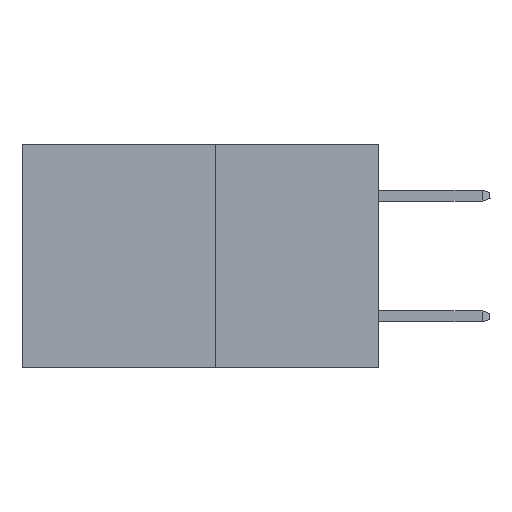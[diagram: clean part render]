
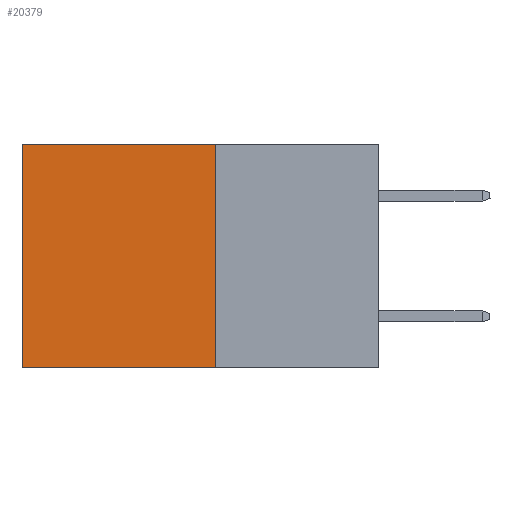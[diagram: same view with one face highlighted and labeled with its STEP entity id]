
A CAD part, left-side view. The second image highlights one B-rep face of the part: STEP entity #20379.
In plain terms, the highlighted planar face has unit normal (-1, 0, 0).
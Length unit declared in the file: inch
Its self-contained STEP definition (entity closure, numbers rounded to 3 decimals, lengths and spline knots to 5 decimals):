
#236 = LINE ( 'NONE', #17223, #17540 ) ;
#738 = ORIENTED_EDGE ( 'NONE', *, *, #6208, .T. ) ;
#1048 = DIRECTION ( 'NONE',  ( 1., 0., 0. ) ) ;
#1437 = CARTESIAN_POINT ( 'NONE',  ( 0.277, 0.59, 0. ) ) ;
#1688 = LINE ( 'NONE', #9182, #18836 ) ;
#2247 = VERTEX_POINT ( 'NONE', #9369 ) ;
#2275 = FACE_OUTER_BOUND ( 'NONE', #19413, .T. ) ;
#2917 = CARTESIAN_POINT ( 'NONE',  ( 0.277, 0.27, -0.37 ) ) ;
#3136 = VERTEX_POINT ( 'NONE', #7592 ) ;
#3161 = ORIENTED_EDGE ( 'NONE', *, *, #16661, .F. ) ;
#4608 = DIRECTION ( 'NONE',  ( 0., 1., 0. ) ) ;
#5179 = VERTEX_POINT ( 'NONE', #1437 ) ;
#6208 = EDGE_CURVE ( 'NONE', #5179, #2247, #236, .T. ) ;
#6467 = EDGE_CURVE ( 'NONE', #13673, #2247, #15794, .T. ) ;
#7592 = CARTESIAN_POINT ( 'NONE',  ( 0.277, 0.27, 0. ) ) ;
#7734 = DIRECTION ( 'NONE',  ( 0., 1., 0. ) ) ;
#8512 = VECTOR ( 'NONE', #4608, 39.37008 ) ;
#9182 = CARTESIAN_POINT ( 'NONE',  ( 0.277, 0.27, -0.37 ) ) ;
#9369 = CARTESIAN_POINT ( 'NONE',  ( 0.277, 0.59, -0.37 ) ) ;
#10660 = DIRECTION ( 'NONE',  ( 0., 0., -1. ) ) ;
#11067 = CARTESIAN_POINT ( 'NONE',  ( 0.277, 0.27, 0. ) ) ;
#11140 = CARTESIAN_POINT ( 'NONE',  ( 0.277, 0.27, -0.37 ) ) ;
#11687 = ORIENTED_EDGE ( 'NONE', *, *, #20364, .T. ) ;
#12481 = AXIS2_PLACEMENT_3D ( 'NONE', #11140, #1048, #12792 ) ;
#12485 = DIRECTION ( 'NONE',  ( 0., 0., -1. ) ) ;
#12792 = DIRECTION ( 'NONE',  ( 0., 0., -1. ) ) ;
#13673 = VERTEX_POINT ( 'NONE', #15403 ) ;
#15403 = CARTESIAN_POINT ( 'NONE',  ( 0.277, 0.27, -0.37 ) ) ;
#15579 = LINE ( 'NONE', #11067, #19352 ) ;
#15794 = LINE ( 'NONE', #2917, #8512 ) ;
#16661 = EDGE_CURVE ( 'NONE', #3136, #13673, #1688, .T. ) ;
#17223 = CARTESIAN_POINT ( 'NONE',  ( 0.277, 0.59, -0.37 ) ) ;
#17540 = VECTOR ( 'NONE', #10660, 39.37008 ) ;
#18836 = VECTOR ( 'NONE', #12485, 39.37008 ) ;
#19352 = VECTOR ( 'NONE', #7734, 39.37008 ) ;
#19413 = EDGE_LOOP ( 'NONE', ( #738, #21325, #3161, #11687 ) ) ;
#20364 = EDGE_CURVE ( 'NONE', #3136, #5179, #15579, .T. ) ;
#20379 = ADVANCED_FACE ( 'NONE', ( #2275 ), #20893, .F. ) ;
#20893 = PLANE ( 'NONE',  #12481 ) ;
#21325 = ORIENTED_EDGE ( 'NONE', *, *, #6467, .F. ) ;
